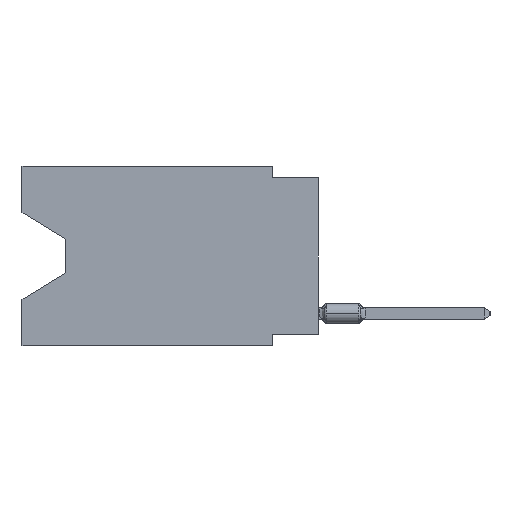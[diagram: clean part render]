
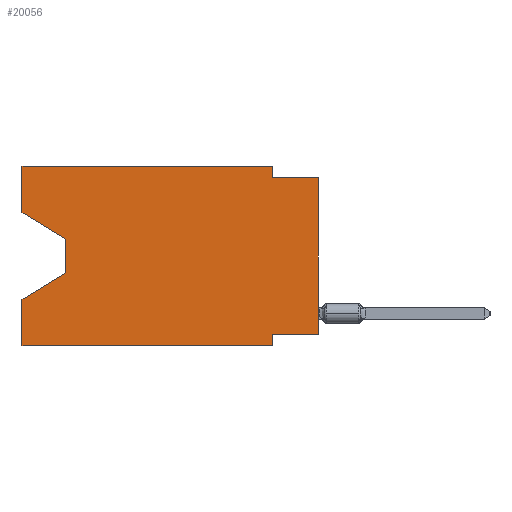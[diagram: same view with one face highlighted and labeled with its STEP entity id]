
A CAD part, left-side view. The second image highlights one B-rep face of the part: STEP entity #20056.
In plain terms, the highlighted planar face has unit normal (-1, 0, 0).
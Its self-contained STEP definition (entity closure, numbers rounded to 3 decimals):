
#1 = CARTESIAN_POINT ( 'NONE',  ( 0., 0., -9.271 ) ) ;
#443 = EDGE_LOOP ( 'NONE', ( #2721, #6788, #22894, #3877, #24732, #30149, #21128, #19308, #1417, #24574, #25473, #19051 ) ) ;
#475 = EDGE_CURVE ( 'NONE', #21589, #22187, #9562, .T. ) ;
#646 = EDGE_CURVE ( 'NONE', #13148, #11335, #7780, .T. ) ;
#1303 = DIRECTION ( 'NONE',  ( 0., 0., 1. ) ) ;
#1417 = ORIENTED_EDGE ( 'NONE', *, *, #30589, .F. ) ;
#1494 = VECTOR ( 'NONE', #30352, 1000. ) ;
#1597 = CARTESIAN_POINT ( 'NONE',  ( 0., 16.383, 0. ) ) ;
#1620 = CARTESIAN_POINT ( 'NONE',  ( 0., 2.54, -9.906 ) ) ;
#2202 = EDGE_CURVE ( 'NONE', #22202, #13300, #11472, .T. ) ;
#2721 = ORIENTED_EDGE ( 'NONE', *, *, #16294, .T. ) ;
#2824 = CARTESIAN_POINT ( 'NONE',  ( 0., 2.54, -0.635 ) ) ;
#3638 = CARTESIAN_POINT ( 'NONE',  ( 0., 16.383, 0. ) ) ;
#3801 = DIRECTION ( 'NONE',  ( 0., -1., 0. ) ) ;
#3877 = ORIENTED_EDGE ( 'NONE', *, *, #26405, .F. ) ;
#3951 = CARTESIAN_POINT ( 'NONE',  ( 0., 16.383, -9.906 ) ) ;
#4696 = CARTESIAN_POINT ( 'NONE',  ( 0., 16.383, 0. ) ) ;
#5582 = EDGE_CURVE ( 'NONE', #22202, #25679, #8390, .T. ) ;
#6719 = DIRECTION ( 'NONE',  ( 0., 0., -1. ) ) ;
#6788 = ORIENTED_EDGE ( 'NONE', *, *, #475, .T. ) ;
#7305 = EDGE_CURVE ( 'NONE', #22187, #15512, #25143, .T. ) ;
#7780 = LINE ( 'NONE', #14431, #10098 ) ;
#8390 = LINE ( 'NONE', #12875, #19935 ) ;
#8806 = VERTEX_POINT ( 'NONE', #24849 ) ;
#8954 = LINE ( 'NONE', #13898, #28120 ) ;
#9043 = DIRECTION ( 'NONE',  ( 1., 0., 0. ) ) ;
#9562 = LINE ( 'NONE', #16688, #30378 ) ;
#9691 = EDGE_CURVE ( 'NONE', #8806, #25505, #8954, .T. ) ;
#10098 = VECTOR ( 'NONE', #14583, 1000. ) ;
#10331 = CARTESIAN_POINT ( 'NONE',  ( 0., 2.54, -9.906 ) ) ;
#10620 = VECTOR ( 'NONE', #29956, 1000. ) ;
#11335 = VERTEX_POINT ( 'NONE', #13278 ) ;
#11472 = LINE ( 'NONE', #1, #1494 ) ;
#11512 = LINE ( 'NONE', #18472, #28863 ) ;
#11618 = CARTESIAN_POINT ( 'NONE',  ( 0., 13.97, -5.893 ) ) ;
#11730 = VECTOR ( 'NONE', #29201, 1000. ) ;
#11953 = DIRECTION ( 'NONE',  ( 0., -0.855, -0.519 ) ) ;
#12743 = VECTOR ( 'NONE', #27771, 1000. ) ;
#12875 = CARTESIAN_POINT ( 'NONE',  ( 0., 0., 0. ) ) ;
#13148 = VERTEX_POINT ( 'NONE', #13662 ) ;
#13278 = CARTESIAN_POINT ( 'NONE',  ( 0., 16.383, 0. ) ) ;
#13300 = VERTEX_POINT ( 'NONE', #19612 ) ;
#13361 = CARTESIAN_POINT ( 'NONE',  ( 0., 13.97, -4.013 ) ) ;
#13662 = CARTESIAN_POINT ( 'NONE',  ( 0., 16.383, -2.546 ) ) ;
#13898 = CARTESIAN_POINT ( 'NONE',  ( 0., 2.54, 0. ) ) ;
#14101 = AXIS2_PLACEMENT_3D ( 'NONE', #4696, #9043, #6719 ) ;
#14431 = CARTESIAN_POINT ( 'NONE',  ( 0., 16.383, 0. ) ) ;
#14583 = DIRECTION ( 'NONE',  ( 0., 0., 1. ) ) ;
#14915 = VECTOR ( 'NONE', #1303, 1000. ) ;
#15428 = VERTEX_POINT ( 'NONE', #24011 ) ;
#15512 = VERTEX_POINT ( 'NONE', #22825 ) ;
#15703 = CARTESIAN_POINT ( 'NONE',  ( 0., 13.97, -5.893 ) ) ;
#16294 = EDGE_CURVE ( 'NONE', #13148, #21589, #11512, .T. ) ;
#16311 = FACE_OUTER_BOUND ( 'NONE', #443, .T. ) ;
#16688 = CARTESIAN_POINT ( 'NONE',  ( 0., 13.97, -4.013 ) ) ;
#16834 = CARTESIAN_POINT ( 'NONE',  ( 0., 0., -0.635 ) ) ;
#17886 = CARTESIAN_POINT ( 'NONE',  ( 0., 0., -0.635 ) ) ;
#18472 = CARTESIAN_POINT ( 'NONE',  ( 0., 16.383, -2.546 ) ) ;
#19051 = ORIENTED_EDGE ( 'NONE', *, *, #646, .F. ) ;
#19308 = ORIENTED_EDGE ( 'NONE', *, *, #5582, .T. ) ;
#19574 = EDGE_CURVE ( 'NONE', #11335, #8806, #26871, .T. ) ;
#19612 = CARTESIAN_POINT ( 'NONE',  ( 0., 2.54, -9.271 ) ) ;
#19935 = VECTOR ( 'NONE', #20158, 1000. ) ;
#20044 = VECTOR ( 'NONE', #29505, 1000. ) ;
#20056 = ADVANCED_FACE ( 'NONE', ( #16311 ), #27925, .F. ) ;
#20158 = DIRECTION ( 'NONE',  ( 0., 0., 1. ) ) ;
#20862 = DIRECTION ( 'NONE',  ( 0., 0., -1. ) ) ;
#21128 = ORIENTED_EDGE ( 'NONE', *, *, #2202, .F. ) ;
#21317 = DIRECTION ( 'NONE',  ( 0., 0., -1. ) ) ;
#21589 = VERTEX_POINT ( 'NONE', #13361 ) ;
#22099 = LINE ( 'NONE', #10331, #11730 ) ;
#22187 = VERTEX_POINT ( 'NONE', #11618 ) ;
#22202 = VERTEX_POINT ( 'NONE', #25554 ) ;
#22229 = LINE ( 'NONE', #3951, #10620 ) ;
#22515 = LINE ( 'NONE', #1597, #14915 ) ;
#22825 = CARTESIAN_POINT ( 'NONE',  ( 0., 16.383, -7.36 ) ) ;
#22894 = ORIENTED_EDGE ( 'NONE', *, *, #7305, .T. ) ;
#23646 = VERTEX_POINT ( 'NONE', #1620 ) ;
#24011 = CARTESIAN_POINT ( 'NONE',  ( 0., 16.383, -9.906 ) ) ;
#24574 = ORIENTED_EDGE ( 'NONE', *, *, #9691, .F. ) ;
#24731 = EDGE_CURVE ( 'NONE', #13300, #23646, #22099, .T. ) ;
#24732 = ORIENTED_EDGE ( 'NONE', *, *, #30527, .T. ) ;
#24849 = CARTESIAN_POINT ( 'NONE',  ( 0., 2.54, 0. ) ) ;
#25143 = LINE ( 'NONE', #15703, #12743 ) ;
#25473 = ORIENTED_EDGE ( 'NONE', *, *, #19574, .F. ) ;
#25505 = VERTEX_POINT ( 'NONE', #2824 ) ;
#25554 = CARTESIAN_POINT ( 'NONE',  ( 0., 0., -9.271 ) ) ;
#25679 = VERTEX_POINT ( 'NONE', #16834 ) ;
#26405 = EDGE_CURVE ( 'NONE', #15428, #15512, #22515, .T. ) ;
#26871 = LINE ( 'NONE', #3638, #20044 ) ;
#27330 = LINE ( 'NONE', #17886, #28351 ) ;
#27771 = DIRECTION ( 'NONE',  ( 0., 0.855, -0.519 ) ) ;
#27925 = PLANE ( 'NONE',  #14101 ) ;
#28120 = VECTOR ( 'NONE', #20862, 1000. ) ;
#28351 = VECTOR ( 'NONE', #3801, 1000. ) ;
#28863 = VECTOR ( 'NONE', #11953, 1000. ) ;
#29201 = DIRECTION ( 'NONE',  ( 0., 0., -1. ) ) ;
#29505 = DIRECTION ( 'NONE',  ( 0., -1., 0. ) ) ;
#29956 = DIRECTION ( 'NONE',  ( 0., -1., 0. ) ) ;
#30149 = ORIENTED_EDGE ( 'NONE', *, *, #24731, .F. ) ;
#30352 = DIRECTION ( 'NONE',  ( 0., 1., 0. ) ) ;
#30378 = VECTOR ( 'NONE', #21317, 1000. ) ;
#30527 = EDGE_CURVE ( 'NONE', #15428, #23646, #22229, .T. ) ;
#30589 = EDGE_CURVE ( 'NONE', #25505, #25679, #27330, .T. ) ;
